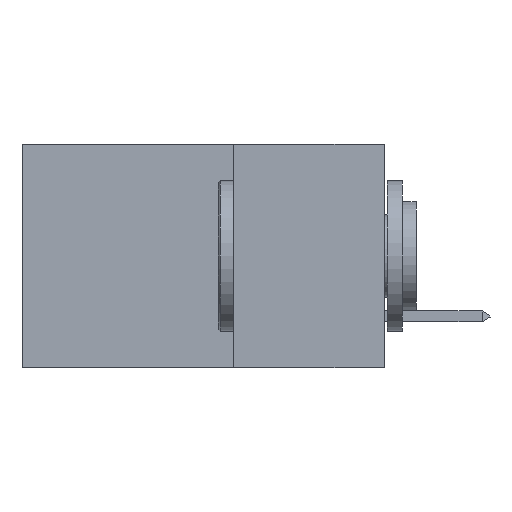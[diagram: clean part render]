
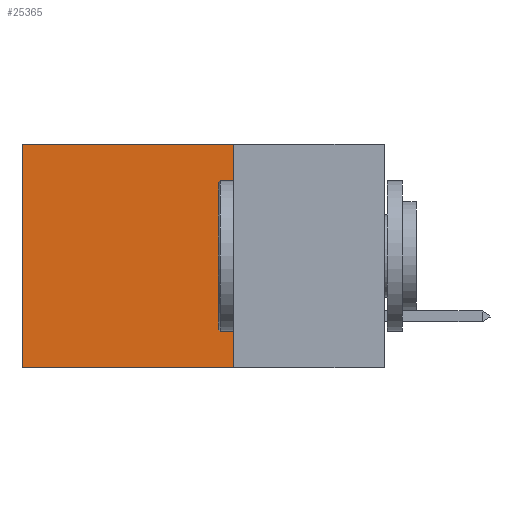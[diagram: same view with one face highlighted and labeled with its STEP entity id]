
A CAD part, left-side view. The second image highlights one B-rep face of the part: STEP entity #25365.
In plain terms, the highlighted planar face has unit normal (-1, 0, 0).
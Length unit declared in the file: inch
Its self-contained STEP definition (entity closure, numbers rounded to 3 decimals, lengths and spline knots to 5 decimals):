
#201 = VECTOR ( 'NONE', #1217, 39.37008 ) ;
#1081 = LINE ( 'NONE', #28438, #12655 ) ;
#1217 = DIRECTION ( 'NONE',  ( 0., 1., 0. ) ) ;
#1541 = CARTESIAN_POINT ( 'NONE',  ( 0.2875, 0.25, -0.37 ) ) ;
#1850 = VERTEX_POINT ( 'NONE', #10911 ) ;
#2113 = DIRECTION ( 'NONE',  ( 0., 0., -1. ) ) ;
#3340 = EDGE_CURVE ( 'NONE', #28704, #4355, #26968, .T. ) ;
#4355 = VERTEX_POINT ( 'NONE', #10407 ) ;
#5807 = VERTEX_POINT ( 'NONE', #35376 ) ;
#10407 = CARTESIAN_POINT ( 'NONE',  ( 0.2875, 0.6, -0.37 ) ) ;
#10911 = CARTESIAN_POINT ( 'NONE',  ( 0.2875, 0.25, 0. ) ) ;
#11221 = LINE ( 'NONE', #1541, #201 ) ;
#11819 = FACE_OUTER_BOUND ( 'NONE', #28927, .T. ) ;
#12655 = VECTOR ( 'NONE', #2113, 39.37008 ) ;
#13152 = VECTOR ( 'NONE', #37018, 39.37008 ) ;
#13939 = ORIENTED_EDGE ( 'NONE', *, *, #3340, .T. ) ;
#15384 = ORIENTED_EDGE ( 'NONE', *, *, #33234, .F. ) ;
#19383 = PLANE ( 'NONE',  #41738 ) ;
#22220 = EDGE_CURVE ( 'NONE', #5807, #4355, #11221, .T. ) ;
#23011 = ORIENTED_EDGE ( 'NONE', *, *, #30940, .T. ) ;
#23012 = ORIENTED_EDGE ( 'NONE', *, *, #22220, .F. ) ;
#25002 = DIRECTION ( 'NONE',  ( 0., 1., 0. ) ) ;
#25365 = ADVANCED_FACE ( 'NONE', ( #11819 ), #19383, .F. ) ;
#25728 = DIRECTION ( 'NONE',  ( 0., 0., -1. ) ) ;
#26968 = LINE ( 'NONE', #27292, #13152 ) ;
#27292 = CARTESIAN_POINT ( 'NONE',  ( 0.2875, 0.6, 0. ) ) ;
#28438 = CARTESIAN_POINT ( 'NONE',  ( 0.2875, 0.25, 0. ) ) ;
#28704 = VERTEX_POINT ( 'NONE', #37155 ) ;
#28927 = EDGE_LOOP ( 'NONE', ( #13939, #23012, #15384, #23011 ) ) ;
#28984 = VECTOR ( 'NONE', #25002, 39.37008 ) ;
#29971 = LINE ( 'NONE', #31403, #28984 ) ;
#30940 = EDGE_CURVE ( 'NONE', #1850, #28704, #29971, .T. ) ;
#31403 = CARTESIAN_POINT ( 'NONE',  ( 0.2875, 0.25, 0. ) ) ;
#32973 = CARTESIAN_POINT ( 'NONE',  ( 0.2875, 0.25, 0. ) ) ;
#33234 = EDGE_CURVE ( 'NONE', #1850, #5807, #1081, .T. ) ;
#35376 = CARTESIAN_POINT ( 'NONE',  ( 0.2875, 0.25, -0.37 ) ) ;
#37018 = DIRECTION ( 'NONE',  ( 0., 0., -1. ) ) ;
#37155 = CARTESIAN_POINT ( 'NONE',  ( 0.2875, 0.6, 0. ) ) ;
#41738 = AXIS2_PLACEMENT_3D ( 'NONE', #32973, #42545, #25728 ) ;
#42545 = DIRECTION ( 'NONE',  ( 1., 0., 0. ) ) ;
